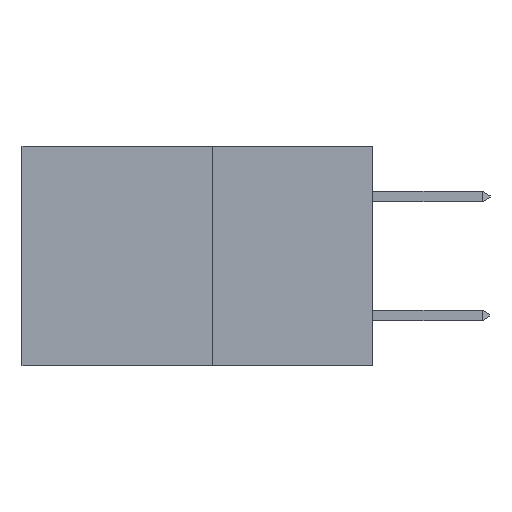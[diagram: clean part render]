
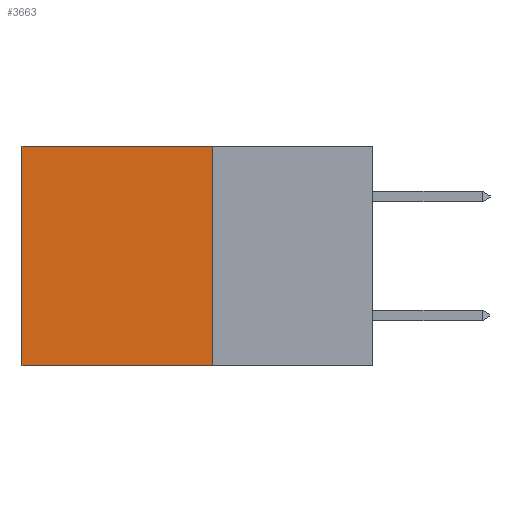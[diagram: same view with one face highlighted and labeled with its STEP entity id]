
A CAD part, left-side view. The second image highlights one B-rep face of the part: STEP entity #3663.
In plain terms, the highlighted planar face has unit normal (-1, 0, 0).
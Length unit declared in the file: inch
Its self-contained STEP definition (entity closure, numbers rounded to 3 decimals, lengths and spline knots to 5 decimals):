
#677 = VECTOR ( 'NONE', #7556, 39.37008 ) ;
#688 = DIRECTION ( 'NONE',  ( 0., 0., -1. ) ) ;
#1148 = CARTESIAN_POINT ( 'NONE',  ( 0.277, 0.59, -0.37 ) ) ;
#1254 = DIRECTION ( 'NONE',  ( 1., 0., 0. ) ) ;
#1599 = VERTEX_POINT ( 'NONE', #4798 ) ;
#1875 = VERTEX_POINT ( 'NONE', #5120 ) ;
#1930 = LINE ( 'NONE', #2796, #6280 ) ;
#1995 = VERTEX_POINT ( 'NONE', #1148 ) ;
#2030 = DIRECTION ( 'NONE',  ( 0., 0., -1. ) ) ;
#2235 = LINE ( 'NONE', #5173, #6600 ) ;
#2796 = CARTESIAN_POINT ( 'NONE',  ( 0.277, 0.59, -0.37 ) ) ;
#3139 = ORIENTED_EDGE ( 'NONE', *, *, #9500, .F. ) ;
#3349 = EDGE_CURVE ( 'NONE', #1599, #9536, #6844, .T. ) ;
#3663 = ADVANCED_FACE ( 'NONE', ( #5375 ), #4232, .F. ) ;
#4131 = CARTESIAN_POINT ( 'NONE',  ( 0.277, 0.59, 0. ) ) ;
#4232 = PLANE ( 'NONE',  #6356 ) ;
#4438 = EDGE_CURVE ( 'NONE', #9536, #1995, #1930, .T. ) ;
#4561 = VECTOR ( 'NONE', #6660, 39.37008 ) ;
#4798 = CARTESIAN_POINT ( 'NONE',  ( 0.277, 0.27, 0. ) ) ;
#5120 = CARTESIAN_POINT ( 'NONE',  ( 0.277, 0.27, -0.37 ) ) ;
#5173 = CARTESIAN_POINT ( 'NONE',  ( 0.277, 0.27, -0.37 ) ) ;
#5375 = FACE_OUTER_BOUND ( 'NONE', #6823, .T. ) ;
#5522 = DIRECTION ( 'NONE',  ( 0., 0., -1. ) ) ;
#5548 = ORIENTED_EDGE ( 'NONE', *, *, #8554, .F. ) ;
#5629 = CARTESIAN_POINT ( 'NONE',  ( 0.277, 0.27, -0.37 ) ) ;
#6280 = VECTOR ( 'NONE', #688, 39.37008 ) ;
#6356 = AXIS2_PLACEMENT_3D ( 'NONE', #5629, #1254, #2030 ) ;
#6600 = VECTOR ( 'NONE', #5522, 39.37008 ) ;
#6660 = DIRECTION ( 'NONE',  ( 0., 1., 0. ) ) ;
#6823 = EDGE_LOOP ( 'NONE', ( #9761, #3139, #5548, #7804 ) ) ;
#6844 = LINE ( 'NONE', #7930, #4561 ) ;
#7556 = DIRECTION ( 'NONE',  ( 0., 1., 0. ) ) ;
#7804 = ORIENTED_EDGE ( 'NONE', *, *, #3349, .T. ) ;
#7930 = CARTESIAN_POINT ( 'NONE',  ( 0.277, 0.27, 0. ) ) ;
#8554 = EDGE_CURVE ( 'NONE', #1599, #1875, #2235, .T. ) ;
#9500 = EDGE_CURVE ( 'NONE', #1875, #1995, #9855, .T. ) ;
#9536 = VERTEX_POINT ( 'NONE', #4131 ) ;
#9761 = ORIENTED_EDGE ( 'NONE', *, *, #4438, .T. ) ;
#9855 = LINE ( 'NONE', #10859, #677 ) ;
#10859 = CARTESIAN_POINT ( 'NONE',  ( 0.277, 0.27, -0.37 ) ) ;
